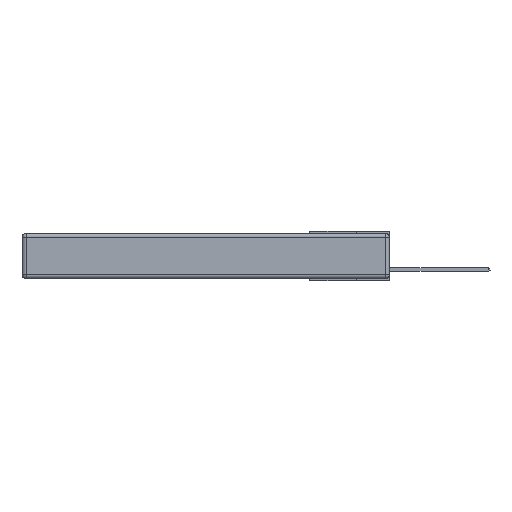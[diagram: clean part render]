
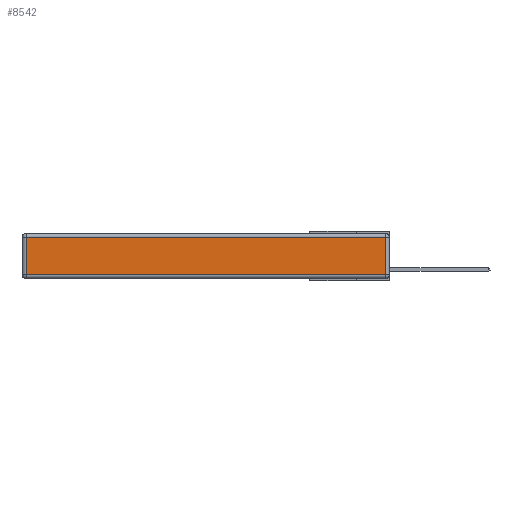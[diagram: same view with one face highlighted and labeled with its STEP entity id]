
A CAD part, left-side view. The second image highlights one B-rep face of the part: STEP entity #8542.
In plain terms, the highlighted planar face has unit normal (-1, 0, 0).
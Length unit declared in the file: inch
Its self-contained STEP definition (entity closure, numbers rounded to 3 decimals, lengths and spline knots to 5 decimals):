
#836 = FACE_OUTER_BOUND ( 'NONE', #23144, .T. ) ;
#904 = EDGE_CURVE ( 'NONE', #20539, #26408, #7897, .T. ) ;
#1353 = DIRECTION ( 'NONE',  ( 0., 0., 1. ) ) ;
#2822 = VECTOR ( 'NONE', #1353, 39.37008 ) ;
#3016 = CARTESIAN_POINT ( 'NONE',  ( 0., 0., -0.313 ) ) ;
#5950 = ORIENTED_EDGE ( 'NONE', *, *, #15894, .T. ) ;
#6179 = LINE ( 'NONE', #12107, #2822 ) ;
#6522 = VECTOR ( 'NONE', #14175, 39.37008 ) ;
#6640 = ORIENTED_EDGE ( 'NONE', *, *, #904, .T. ) ;
#7775 = LINE ( 'NONE', #3016, #21603 ) ;
#7897 = LINE ( 'NONE', #26822, #6522 ) ;
#7986 = AXIS2_PLACEMENT_3D ( 'NONE', #22769, #16380, #14854 ) ;
#8515 = CARTESIAN_POINT ( 'NONE',  ( 0., 0.03, -0.03 ) ) ;
#8542 = ADVANCED_FACE ( 'NONE', ( #836 ), #20610, .T. ) ;
#8749 = CARTESIAN_POINT ( 'NONE',  ( 0., 2.72, -0.313 ) ) ;
#9038 = CARTESIAN_POINT ( 'NONE',  ( 0., 2.72, -0.03 ) ) ;
#10059 = VERTEX_POINT ( 'NONE', #25397 ) ;
#10324 = EDGE_CURVE ( 'NONE', #13893, #20539, #23626, .T. ) ;
#10763 = ORIENTED_EDGE ( 'NONE', *, *, #10324, .T. ) ;
#12107 = CARTESIAN_POINT ( 'NONE',  ( 0., 0.03, -0.343 ) ) ;
#13893 = VERTEX_POINT ( 'NONE', #8515 ) ;
#14175 = DIRECTION ( 'NONE',  ( 0., 0., -1. ) ) ;
#14317 = CARTESIAN_POINT ( 'NONE',  ( 0., 2.75, -0.03 ) ) ;
#14854 = DIRECTION ( 'NONE',  ( 0., 0., 1. ) ) ;
#15894 = EDGE_CURVE ( 'NONE', #26408, #10059, #7775, .T. ) ;
#16380 = DIRECTION ( 'NONE',  ( -1., 0., 0. ) ) ;
#18778 = ORIENTED_EDGE ( 'NONE', *, *, #20701, .T. ) ;
#18993 = DIRECTION ( 'NONE',  ( 0., 1., 0. ) ) ;
#20539 = VERTEX_POINT ( 'NONE', #9038 ) ;
#20610 = PLANE ( 'NONE',  #7986 ) ;
#20701 = EDGE_CURVE ( 'NONE', #10059, #13893, #6179, .T. ) ;
#21603 = VECTOR ( 'NONE', #24293, 39.37008 ) ;
#22769 = CARTESIAN_POINT ( 'NONE',  ( 0., 0., -0.343 ) ) ;
#23144 = EDGE_LOOP ( 'NONE', ( #5950, #18778, #10763, #6640 ) ) ;
#23626 = LINE ( 'NONE', #14317, #23947 ) ;
#23947 = VECTOR ( 'NONE', #18993, 39.37008 ) ;
#24293 = DIRECTION ( 'NONE',  ( 0., -1., 0. ) ) ;
#25397 = CARTESIAN_POINT ( 'NONE',  ( 0., 0.03, -0.313 ) ) ;
#26408 = VERTEX_POINT ( 'NONE', #8749 ) ;
#26822 = CARTESIAN_POINT ( 'NONE',  ( 0., 2.72, -0.343 ) ) ;
